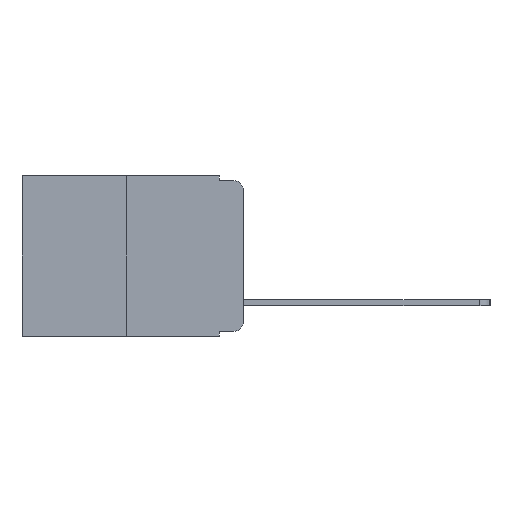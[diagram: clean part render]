
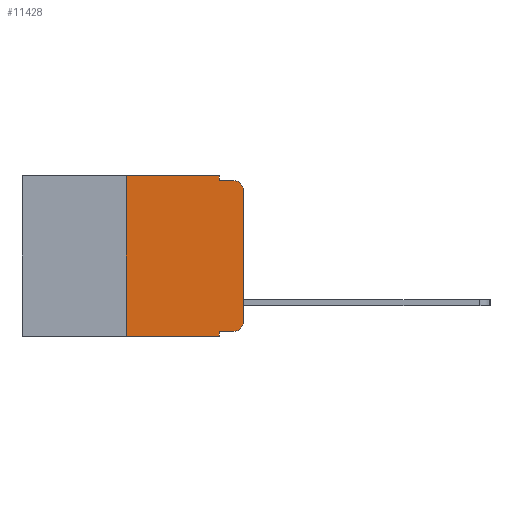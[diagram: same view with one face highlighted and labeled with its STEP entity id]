
A CAD part, left-side view. The second image highlights one B-rep face of the part: STEP entity #11428.
In plain terms, the highlighted planar face has unit normal (-1, 0, 0).
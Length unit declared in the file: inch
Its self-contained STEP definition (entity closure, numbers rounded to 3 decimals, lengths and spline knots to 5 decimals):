
#293 = LINE ( 'NONE', #10761, #14706 ) ;
#331 = ORIENTED_EDGE ( 'NONE', *, *, #14374, .T. ) ;
#796 = AXIS2_PLACEMENT_3D ( 'NONE', #10883, #2605, #12228 ) ;
#907 = DIRECTION ( 'NONE',  ( 0., 0., -1. ) ) ;
#1113 = VERTEX_POINT ( 'NONE', #1505 ) ;
#1381 = CARTESIAN_POINT ( 'NONE',  ( 0., 0.051, -0.01 ) ) ;
#1505 = CARTESIAN_POINT ( 'NONE',  ( 0., 0.02, -0.333 ) ) ;
#1778 = PLANE ( 'NONE',  #13250 ) ;
#1798 = VECTOR ( 'NONE', #3420, 39.37008 ) ;
#2313 = ORIENTED_EDGE ( 'NONE', *, *, #7794, .T. ) ;
#2504 = ORIENTED_EDGE ( 'NONE', *, *, #3510, .F. ) ;
#2605 = DIRECTION ( 'NONE',  ( -1., 0., 0. ) ) ;
#2698 = CARTESIAN_POINT ( 'NONE',  ( 0., 0.25, -0.343 ) ) ;
#2879 = EDGE_CURVE ( 'NONE', #14754, #5811, #15952, .T. ) ;
#3026 = LINE ( 'NONE', #4353, #17059 ) ;
#3253 = DIRECTION ( 'NONE',  ( 0., 0., -1. ) ) ;
#3316 = CARTESIAN_POINT ( 'NONE',  ( 0., 0.051, -0.333 ) ) ;
#3420 = DIRECTION ( 'NONE',  ( 0., 0., -1. ) ) ;
#3430 = CIRCLE ( 'NONE', #12657, 0.02 ) ;
#3510 = EDGE_CURVE ( 'NONE', #3765, #13872, #15732, .T. ) ;
#3741 = DIRECTION ( 'NONE',  ( 0., -1., 0. ) ) ;
#3765 = VERTEX_POINT ( 'NONE', #4639 ) ;
#3836 = ORIENTED_EDGE ( 'NONE', *, *, #14026, .T. ) ;
#4353 = CARTESIAN_POINT ( 'NONE',  ( 0., 0.473, -0.343 ) ) ;
#4639 = CARTESIAN_POINT ( 'NONE',  ( 0., 0.051, 0. ) ) ;
#5135 = EDGE_LOOP ( 'NONE', ( #9280, #2313, #9700, #2504, #6220, #6658, #13889, #17386, #3836, #331 ) ) ;
#5407 = LINE ( 'NONE', #12287, #15819 ) ;
#5416 = VECTOR ( 'NONE', #3741, 39.37008 ) ;
#5470 = DIRECTION ( 'NONE',  ( 0., 0., 1. ) ) ;
#5811 = VERTEX_POINT ( 'NONE', #6600 ) ;
#6220 = ORIENTED_EDGE ( 'NONE', *, *, #15137, .F. ) ;
#6317 = CARTESIAN_POINT ( 'NONE',  ( 0., 0.051, 0. ) ) ;
#6597 = CARTESIAN_POINT ( 'NONE',  ( 0., 0., -0.03 ) ) ;
#6600 = CARTESIAN_POINT ( 'NONE',  ( 0., 0.051, -0.343 ) ) ;
#6658 = ORIENTED_EDGE ( 'NONE', *, *, #16585, .F. ) ;
#6917 = DIRECTION ( 'NONE',  ( 0., -1., 0. ) ) ;
#7794 = EDGE_CURVE ( 'NONE', #13631, #11183, #3430, .T. ) ;
#7798 = LINE ( 'NONE', #3316, #15410 ) ;
#7972 = CARTESIAN_POINT ( 'NONE',  ( 0., 0.02, -0.01 ) ) ;
#8545 = VECTOR ( 'NONE', #10287, 39.37008 ) ;
#9036 = VERTEX_POINT ( 'NONE', #2698 ) ;
#9280 = ORIENTED_EDGE ( 'NONE', *, *, #14399, .T. ) ;
#9351 = DIRECTION ( 'NONE',  ( -1., 0., 0. ) ) ;
#9631 = EDGE_CURVE ( 'NONE', #13872, #11183, #12252, .T. ) ;
#9697 = LINE ( 'NONE', #17658, #15589 ) ;
#9700 = ORIENTED_EDGE ( 'NONE', *, *, #9631, .F. ) ;
#10241 = CARTESIAN_POINT ( 'NONE',  ( 0., 0.25, 0. ) ) ;
#10287 = DIRECTION ( 'NONE',  ( 0., 0., -1. ) ) ;
#10678 = CARTESIAN_POINT ( 'NONE',  ( 0., 0.051, -0.01 ) ) ;
#10761 = CARTESIAN_POINT ( 'NONE',  ( 0., 0.25, 0. ) ) ;
#10883 = CARTESIAN_POINT ( 'NONE',  ( 0., 0.02, -0.313 ) ) ;
#11183 = VERTEX_POINT ( 'NONE', #7972 ) ;
#11428 = ADVANCED_FACE ( 'NONE', ( #15784 ), #1778, .F. ) ;
#11474 = VERTEX_POINT ( 'NONE', #10241 ) ;
#11476 = DIRECTION ( 'NONE',  ( 1., 0., 0. ) ) ;
#11639 = CARTESIAN_POINT ( 'NONE',  ( 0., 0.051, 0. ) ) ;
#12228 = DIRECTION ( 'NONE',  ( 0., 0., -1. ) ) ;
#12252 = LINE ( 'NONE', #10678, #5416 ) ;
#12287 = CARTESIAN_POINT ( 'NONE',  ( 0., 0., 0. ) ) ;
#12657 = AXIS2_PLACEMENT_3D ( 'NONE', #17342, #9351, #907 ) ;
#12904 = DIRECTION ( 'NONE',  ( 0., -1., 0. ) ) ;
#13250 = AXIS2_PLACEMENT_3D ( 'NONE', #14138, #11476, #3253 ) ;
#13571 = CARTESIAN_POINT ( 'NONE',  ( 0., 0., -0.313 ) ) ;
#13631 = VERTEX_POINT ( 'NONE', #6597 ) ;
#13709 = VERTEX_POINT ( 'NONE', #13571 ) ;
#13872 = VERTEX_POINT ( 'NONE', #1381 ) ;
#13882 = EDGE_CURVE ( 'NONE', #9036, #5811, #3026, .T. ) ;
#13889 = ORIENTED_EDGE ( 'NONE', *, *, #13882, .T. ) ;
#14026 = EDGE_CURVE ( 'NONE', #14754, #1113, #7798, .T. ) ;
#14138 = CARTESIAN_POINT ( 'NONE',  ( 0., 0.473, 0. ) ) ;
#14362 = CARTESIAN_POINT ( 'NONE',  ( 0., 0.051, -0.333 ) ) ;
#14374 = EDGE_CURVE ( 'NONE', #1113, #13709, #16630, .T. ) ;
#14399 = EDGE_CURVE ( 'NONE', #13709, #13631, #5407, .T. ) ;
#14706 = VECTOR ( 'NONE', #16117, 39.37008 ) ;
#14754 = VERTEX_POINT ( 'NONE', #14362 ) ;
#15137 = EDGE_CURVE ( 'NONE', #11474, #3765, #9697, .T. ) ;
#15410 = VECTOR ( 'NONE', #12904, 39.37008 ) ;
#15589 = VECTOR ( 'NONE', #6917, 39.37008 ) ;
#15732 = LINE ( 'NONE', #11639, #8545 ) ;
#15784 = FACE_OUTER_BOUND ( 'NONE', #5135, .T. ) ;
#15819 = VECTOR ( 'NONE', #5470, 39.37008 ) ;
#15952 = LINE ( 'NONE', #6317, #1798 ) ;
#16117 = DIRECTION ( 'NONE',  ( 0., 0., 1. ) ) ;
#16562 = DIRECTION ( 'NONE',  ( 0., -1., 0. ) ) ;
#16585 = EDGE_CURVE ( 'NONE', #9036, #11474, #293, .T. ) ;
#16630 = CIRCLE ( 'NONE', #796, 0.02 ) ;
#17059 = VECTOR ( 'NONE', #16562, 39.37008 ) ;
#17342 = CARTESIAN_POINT ( 'NONE',  ( 0., 0.02, -0.03 ) ) ;
#17386 = ORIENTED_EDGE ( 'NONE', *, *, #2879, .F. ) ;
#17658 = CARTESIAN_POINT ( 'NONE',  ( 0., 0.473, 0. ) ) ;
